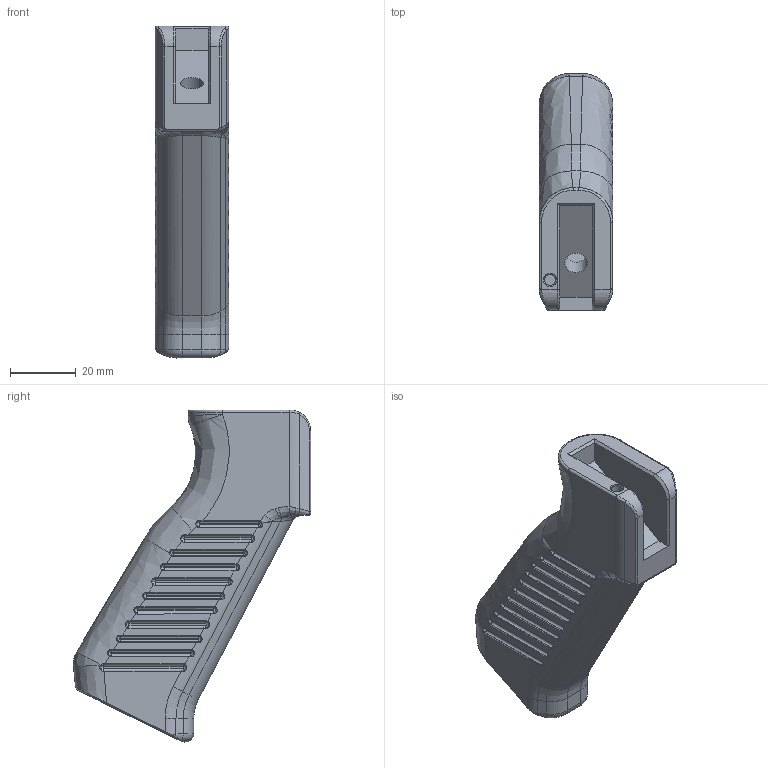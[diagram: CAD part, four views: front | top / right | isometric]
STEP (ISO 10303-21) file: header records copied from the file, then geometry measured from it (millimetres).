
FILE_DESCRIPTION(/* description */ (''),/* implementation_level */ '2;1');
FILE_NAME(/* name */ 'Industrial Grip.step',/* time_stamp */ '2021-10-17T22:58:36-04:00',/* author */ (''),/* organization */ (''),/* preprocessor_version */ 'ST-DEVELOPER v18.1',/* originating_system */ 'Autodesk Translation Framework v10.10.0.1391',/* authorisation */ '');
FILE_SCHEMA (('AUTOMOTIVE_DESIGN { 1 0 10303 214 3 1 1 }'));
Length unit declared in the file: millimetre
Products named in the file (1): Industrial Grip
Bounding box: 22.33 x 72.09 x 100.86 mm (x, y, z)
Volume: 46832.5 mm3; surface area: 19081.3 mm2
Topology: 1 solids, 1 shells, 803 faces, 1877 edges, 1072 vertices
Faces by surface type: bspline 338, cylinder 241, plane 138, torus 78, cone 8
Full cylindrical faces by diameter (mm): 3.4 x1, 6.8 x1, 11.616 x1, 13.416 x1
Entity records: 30158 total; most frequent: CARTESIAN_POINT 13497, ORIENTED_EDGE 3734, DIRECTION 3104, EDGE_CURVE 1867, AXIS2_PLACEMENT_3D 1311, VERTEX_POINT 1072, EDGE_LOOP 811, FACE_OUTER_BOUND 803
